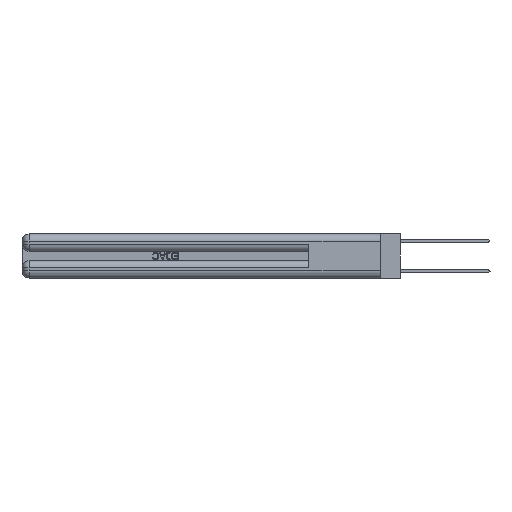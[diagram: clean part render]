
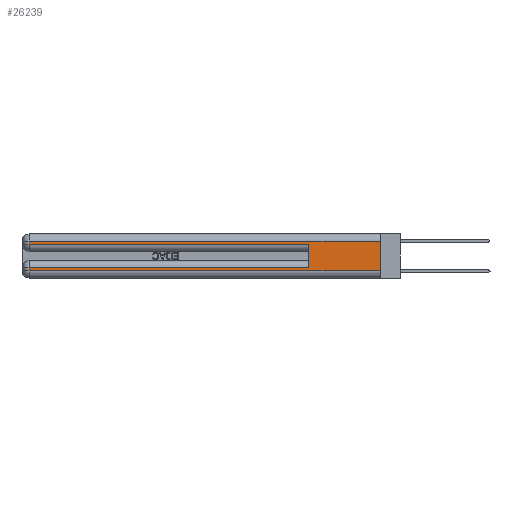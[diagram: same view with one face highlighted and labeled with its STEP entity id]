
A CAD part, left-side view. The second image highlights one B-rep face of the part: STEP entity #26239.
In plain terms, the highlighted planar face has unit normal (-1, 0, 0).
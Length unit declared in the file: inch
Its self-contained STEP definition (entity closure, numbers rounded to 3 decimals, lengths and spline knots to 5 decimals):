
#378 = ORIENTED_EDGE ( 'NONE', *, *, #22414, .T. ) ;
#895 = DIRECTION ( 'NONE',  ( 0., 0., -1. ) ) ;
#1184 = EDGE_CURVE ( 'NONE', #6049, #27302, #26160, .T. ) ;
#2473 = VECTOR ( 'NONE', #19088, 39.37008 ) ;
#4418 = CARTESIAN_POINT ( 'NONE',  ( 0., 0.6, 0.285 ) ) ;
#4563 = CARTESIAN_POINT ( 'NONE',  ( 0., 0., 0.31 ) ) ;
#4751 = ORIENTED_EDGE ( 'NONE', *, *, #23505, .F. ) ;
#4971 = VECTOR ( 'NONE', #23108, 39.37008 ) ;
#5124 = ORIENTED_EDGE ( 'NONE', *, *, #24117, .T. ) ;
#6049 = VERTEX_POINT ( 'NONE', #17279 ) ;
#6214 = DIRECTION ( 'NONE',  ( 0., 0., 1. ) ) ;
#6234 = CARTESIAN_POINT ( 'NONE',  ( 0., 0., 0.06 ) ) ;
#7656 = LINE ( 'NONE', #6234, #19370 ) ;
#8406 = DIRECTION ( 'NONE',  ( 0., 1., 0. ) ) ;
#8787 = ORIENTED_EDGE ( 'NONE', *, *, #17293, .T. ) ;
#9866 = VECTOR ( 'NONE', #20927, 39.37008 ) ;
#10010 = EDGE_CURVE ( 'NONE', #22301, #27302, #19030, .T. ) ;
#10188 = PLANE ( 'NONE',  #26722 ) ;
#10398 = VECTOR ( 'NONE', #8406, 39.37008 ) ;
#12397 = ORIENTED_EDGE ( 'NONE', *, *, #29560, .T. ) ;
#13331 = LINE ( 'NONE', #15685, #25749 ) ;
#13437 = EDGE_LOOP ( 'NONE', ( #4751, #23381, #12397, #21592, #16824, #5124, #378, #8787 ) ) ;
#13529 = VECTOR ( 'NONE', #13605, 39.37008 ) ;
#13605 = DIRECTION ( 'NONE',  ( 0., -1., 0. ) ) ;
#14857 = DIRECTION ( 'NONE',  ( 1., 0., 0. ) ) ;
#14859 = LINE ( 'NONE', #16739, #2473 ) ;
#15334 = LINE ( 'NONE', #4563, #9866 ) ;
#15563 = CARTESIAN_POINT ( 'NONE',  ( 0., 0., 0.31 ) ) ;
#15685 = CARTESIAN_POINT ( 'NONE',  ( 0., 0., 0.37 ) ) ;
#16739 = CARTESIAN_POINT ( 'NONE',  ( 0., 2.94, 0.37 ) ) ;
#16824 = ORIENTED_EDGE ( 'NONE', *, *, #1184, .F. ) ;
#17279 = CARTESIAN_POINT ( 'NONE',  ( 0., 0.6, 0.085 ) ) ;
#17293 = EDGE_CURVE ( 'NONE', #29131, #27929, #7656, .T. ) ;
#19030 = LINE ( 'NONE', #20576, #13529 ) ;
#19088 = DIRECTION ( 'NONE',  ( 0., 0., -1. ) ) ;
#19107 = VERTEX_POINT ( 'NONE', #20793 ) ;
#19370 = VECTOR ( 'NONE', #27218, 39.37008 ) ;
#19664 = VERTEX_POINT ( 'NONE', #20651 ) ;
#20081 = CARTESIAN_POINT ( 'NONE',  ( 0., 0., 0.085 ) ) ;
#20296 = EDGE_CURVE ( 'NONE', #26459, #19107, #15334, .T. ) ;
#20576 = CARTESIAN_POINT ( 'NONE',  ( 0., 0., 0.285 ) ) ;
#20651 = CARTESIAN_POINT ( 'NONE',  ( 0., 2.94, 0.085 ) ) ;
#20793 = CARTESIAN_POINT ( 'NONE',  ( 0., 2.94, 0.31 ) ) ;
#20927 = DIRECTION ( 'NONE',  ( 0., 1., 0. ) ) ;
#21088 = CARTESIAN_POINT ( 'NONE',  ( 0., 2.94, 0.37 ) ) ;
#21324 = FACE_OUTER_BOUND ( 'NONE', #13437, .T. ) ;
#21592 = ORIENTED_EDGE ( 'NONE', *, *, #10010, .T. ) ;
#22301 = VERTEX_POINT ( 'NONE', #22707 ) ;
#22414 = EDGE_CURVE ( 'NONE', #19664, #29131, #29004, .T. ) ;
#22570 = CARTESIAN_POINT ( 'NONE',  ( 0., 0.6, 0.145 ) ) ;
#22707 = CARTESIAN_POINT ( 'NONE',  ( 0., 2.94, 0.285 ) ) ;
#23108 = DIRECTION ( 'NONE',  ( 0., 0., -1. ) ) ;
#23381 = ORIENTED_EDGE ( 'NONE', *, *, #20296, .T. ) ;
#23505 = EDGE_CURVE ( 'NONE', #26459, #27929, #13331, .T. ) ;
#24062 = CARTESIAN_POINT ( 'NONE',  ( 0., 0., 0.06 ) ) ;
#24092 = CARTESIAN_POINT ( 'NONE',  ( 0., 2.94, 0.06 ) ) ;
#24117 = EDGE_CURVE ( 'NONE', #6049, #19664, #28223, .T. ) ;
#25749 = VECTOR ( 'NONE', #29615, 39.37008 ) ;
#26160 = LINE ( 'NONE', #22570, #26889 ) ;
#26239 = ADVANCED_FACE ( 'NONE', ( #21324 ), #10188, .F. ) ;
#26459 = VERTEX_POINT ( 'NONE', #15563 ) ;
#26722 = AXIS2_PLACEMENT_3D ( 'NONE', #28789, #14857, #895 ) ;
#26889 = VECTOR ( 'NONE', #6214, 39.37008 ) ;
#27218 = DIRECTION ( 'NONE',  ( 0., -1., 0. ) ) ;
#27302 = VERTEX_POINT ( 'NONE', #4418 ) ;
#27929 = VERTEX_POINT ( 'NONE', #24062 ) ;
#28223 = LINE ( 'NONE', #20081, #10398 ) ;
#28789 = CARTESIAN_POINT ( 'NONE',  ( 0., 0., 0.37 ) ) ;
#29004 = LINE ( 'NONE', #21088, #4971 ) ;
#29131 = VERTEX_POINT ( 'NONE', #24092 ) ;
#29560 = EDGE_CURVE ( 'NONE', #19107, #22301, #14859, .T. ) ;
#29615 = DIRECTION ( 'NONE',  ( 0., 0., -1. ) ) ;
